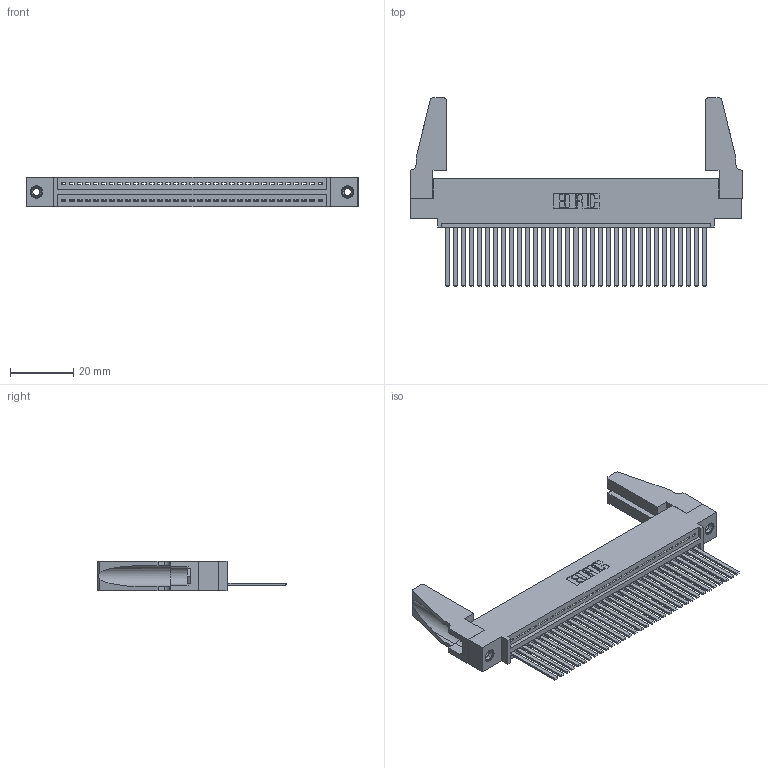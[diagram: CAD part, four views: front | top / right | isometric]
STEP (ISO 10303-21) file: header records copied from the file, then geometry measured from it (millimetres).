
FILE_DESCRIPTION (( 'STEP AP203' ), '1' );
FILE_NAME ('345-033-544-488.STEP', '2019-10-07T16:50:20', ( '' ), ( '' ), 'SwSTEP 2.0', 'SolidWorks 2016', '' );
FILE_SCHEMA (( 'CONFIG_CONTROL_DESIGN' ));
Length unit declared in the file: inch
Products named in the file (5): 345-033-544-488; 345-250-001_345-250-001-102; 345 Part_0.110 Offset - 0.156 Dia-TH; 345-292-001_345-293-144; 345-220-078_345-220-088
Assembly tree (38 placements, depth 2):
  345-033-544-488
    345 Part_0.110 Offset - 0.156 Dia-TH
    345-292-001_345-293-144  x33
    345-250-001_345-250-001-102  x2
    345-220-078_345-220-088  x2
Bounding box: 105.05 x 59.61 x 9.4 mm (x, y, z)
Volume: 13465.8 mm3; surface area: 17808.7 mm2
Topology: 38 solids, 38 shells, 1970 faces, 5881 edges, 3866 vertices
Faces by surface type: plane 1344, cylinder 610, cone 12, torus 4
Entity records: 28144 total; most frequent: CARTESIAN_POINT 4865, ORIENTED_EDGE 4792, DIRECTION 4266, EDGE_CURVE 2396, VECTOR 2094, LINE 2094, VERTEX_POINT 1590, AXIS2_PLACEMENT_3D 1086
